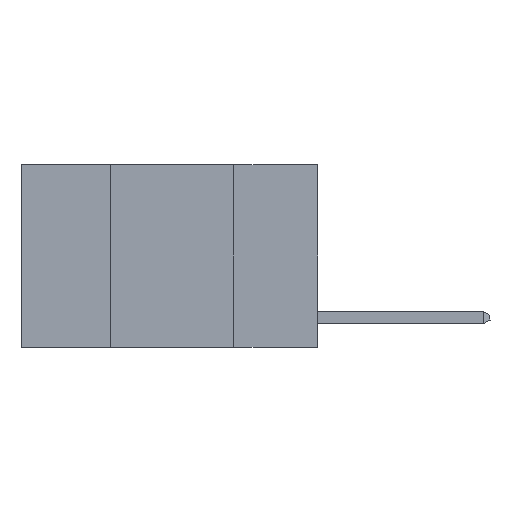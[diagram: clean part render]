
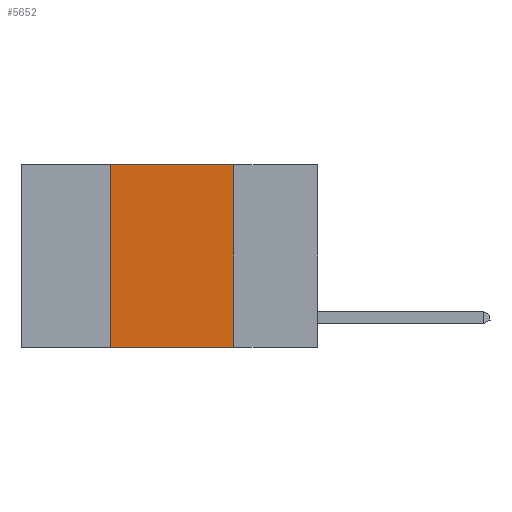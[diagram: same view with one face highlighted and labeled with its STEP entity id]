
A CAD part, left-side view. The second image highlights one B-rep face of the part: STEP entity #5652.
In plain terms, the highlighted planar face has unit normal (-1, 0, 0).
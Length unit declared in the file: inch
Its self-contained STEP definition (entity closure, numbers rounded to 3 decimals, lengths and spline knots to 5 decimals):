
#202 = CARTESIAN_POINT ( 'NONE',  ( 0., 0.42, -0.37 ) ) ;
#726 = ORIENTED_EDGE ( 'NONE', *, *, #2450, .F. ) ;
#1594 = DIRECTION ( 'NONE',  ( 0., 0., 1. ) ) ;
#1700 = CARTESIAN_POINT ( 'NONE',  ( 0., 0.42, 0. ) ) ;
#1879 = CARTESIAN_POINT ( 'NONE',  ( 0., 0.6, 0. ) ) ;
#2450 = EDGE_CURVE ( 'NONE', #20291, #3369, #5553, .T. ) ;
#3075 = EDGE_CURVE ( 'NONE', #3369, #5411, #5253, .T. ) ;
#3369 = VERTEX_POINT ( 'NONE', #7963 ) ;
#4122 = EDGE_CURVE ( 'NONE', #5411, #7185, #20821, .T. ) ;
#4333 = CARTESIAN_POINT ( 'NONE',  ( 0., 0.6, -0.37 ) ) ;
#4705 = VECTOR ( 'NONE', #12292, 39.37008 ) ;
#5253 = LINE ( 'NONE', #1879, #4705 ) ;
#5411 = VERTEX_POINT ( 'NONE', #10125 ) ;
#5553 = LINE ( 'NONE', #1700, #18218 ) ;
#5652 = ADVANCED_FACE ( 'NONE', ( #21043 ), #7564, .F. ) ;
#7185 = VERTEX_POINT ( 'NONE', #22168 ) ;
#7437 = EDGE_LOOP ( 'NONE', ( #13512, #18033, #726, #9985 ) ) ;
#7564 = PLANE ( 'NONE',  #21850 ) ;
#7963 = CARTESIAN_POINT ( 'NONE',  ( 0., 0.42, 0. ) ) ;
#8460 = VECTOR ( 'NONE', #14683, 39.37008 ) ;
#9297 = DIRECTION ( 'NONE',  ( 0., 0., -1. ) ) ;
#9985 = ORIENTED_EDGE ( 'NONE', *, *, #16051, .T. ) ;
#10125 = CARTESIAN_POINT ( 'NONE',  ( 0., 0.17, 0. ) ) ;
#11187 = VECTOR ( 'NONE', #14994, 39.37008 ) ;
#12292 = DIRECTION ( 'NONE',  ( 0., -1., 0. ) ) ;
#13299 = CARTESIAN_POINT ( 'NONE',  ( 0., 0.17, 0. ) ) ;
#13512 = ORIENTED_EDGE ( 'NONE', *, *, #4122, .F. ) ;
#14683 = DIRECTION ( 'NONE',  ( 0., -1., 0. ) ) ;
#14994 = DIRECTION ( 'NONE',  ( 0., 0., -1. ) ) ;
#16051 = EDGE_CURVE ( 'NONE', #20291, #7185, #21584, .T. ) ;
#17847 = CARTESIAN_POINT ( 'NONE',  ( 0., 0.6, 0. ) ) ;
#18033 = ORIENTED_EDGE ( 'NONE', *, *, #3075, .F. ) ;
#18218 = VECTOR ( 'NONE', #1594, 39.37008 ) ;
#19572 = DIRECTION ( 'NONE',  ( 1., 0., 0. ) ) ;
#20291 = VERTEX_POINT ( 'NONE', #202 ) ;
#20821 = LINE ( 'NONE', #13299, #11187 ) ;
#21043 = FACE_OUTER_BOUND ( 'NONE', #7437, .T. ) ;
#21584 = LINE ( 'NONE', #4333, #8460 ) ;
#21850 = AXIS2_PLACEMENT_3D ( 'NONE', #17847, #19572, #9297 ) ;
#22168 = CARTESIAN_POINT ( 'NONE',  ( 0., 0.17, -0.37 ) ) ;
